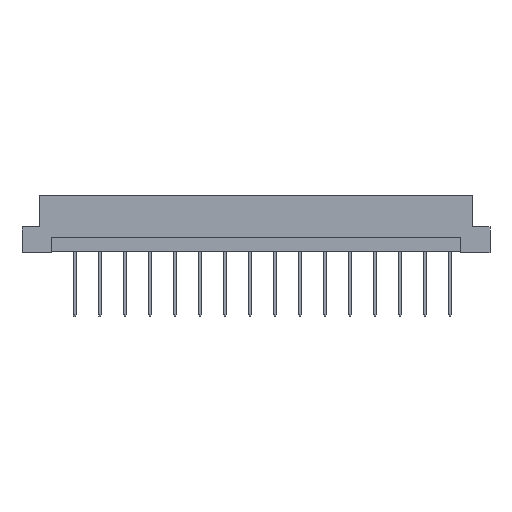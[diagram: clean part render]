
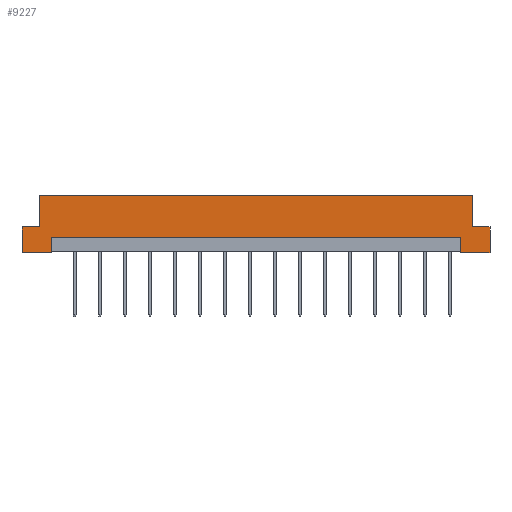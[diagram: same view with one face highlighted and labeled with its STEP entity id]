
A CAD part, front view. The second image highlights one B-rep face of the part: STEP entity #9227.
In plain terms, the highlighted planar face has unit normal (0, -1, 0).
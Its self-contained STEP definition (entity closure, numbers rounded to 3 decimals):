
#10 = VECTOR ( 'NONE', #4077, 1000. ) ;
#165 = VECTOR ( 'NONE', #2074, 1000. ) ;
#184 = CARTESIAN_POINT ( 'NONE',  ( 47.5, -4.3, 11.6 ) ) ;
#233 = VERTEX_POINT ( 'NONE', #4532 ) ;
#282 = EDGE_LOOP ( 'NONE', ( #6928, #5848, #4590, #3941, #6596, #9428, #8726, #10331, #349, #11098, #11080, #9771 ) ) ;
#314 = DIRECTION ( 'NONE',  ( 0., 0., -1. ) ) ;
#349 = ORIENTED_EDGE ( 'NONE', *, *, #6792, .F. ) ;
#429 = CARTESIAN_POINT ( 'NONE',  ( -41.6, -4.3, 0.2 ) ) ;
#440 = VERTEX_POINT ( 'NONE', #8201 ) ;
#538 = CARTESIAN_POINT ( 'NONE',  ( 41.6, -4.3, 0.2 ) ) ;
#577 = CARTESIAN_POINT ( 'NONE',  ( -44., -4.3, 5.2 ) ) ;
#586 = CARTESIAN_POINT ( 'NONE',  ( 47.5, -4.3, 11.6 ) ) ;
#843 = CARTESIAN_POINT ( 'NONE',  ( -47.5, -4.3, 0. ) ) ;
#1109 = DIRECTION ( 'NONE',  ( 1., 0., 0. ) ) ;
#1149 = CARTESIAN_POINT ( 'NONE',  ( 44., -4.3, 5.2 ) ) ;
#1509 = LINE ( 'NONE', #538, #3602 ) ;
#1613 = VERTEX_POINT ( 'NONE', #6684 ) ;
#1621 = VECTOR ( 'NONE', #2677, 1000. ) ;
#2074 = DIRECTION ( 'NONE',  ( 0., 0., -1. ) ) ;
#2199 = LINE ( 'NONE', #586, #10 ) ;
#2232 = CARTESIAN_POINT ( 'NONE',  ( 47.5, -4.3, 11.6 ) ) ;
#2236 = EDGE_CURVE ( 'NONE', #2378, #440, #11209, .T. ) ;
#2378 = VERTEX_POINT ( 'NONE', #7306 ) ;
#2518 = VECTOR ( 'NONE', #5658, 1000. ) ;
#2624 = VECTOR ( 'NONE', #4190, 1000. ) ;
#2677 = DIRECTION ( 'NONE',  ( 1., 0., 0. ) ) ;
#2834 = PLANE ( 'NONE',  #3171 ) ;
#2908 = LINE ( 'NONE', #429, #9891 ) ;
#3005 = DIRECTION ( 'NONE',  ( 0., 1., 0. ) ) ;
#3020 = VECTOR ( 'NONE', #5967, 1000. ) ;
#3037 = LINE ( 'NONE', #6526, #2518 ) ;
#3171 = AXIS2_PLACEMENT_3D ( 'NONE', #184, #3005, #5567 ) ;
#3565 = CARTESIAN_POINT ( 'NONE',  ( -41.6, -4.3, 3. ) ) ;
#3579 = VERTEX_POINT ( 'NONE', #4504 ) ;
#3602 = VECTOR ( 'NONE', #4996, 1000. ) ;
#3723 = VERTEX_POINT ( 'NONE', #4557 ) ;
#3771 = EDGE_CURVE ( 'NONE', #3579, #233, #2908, .T. ) ;
#3941 = ORIENTED_EDGE ( 'NONE', *, *, #4196, .F. ) ;
#4077 = DIRECTION ( 'NONE',  ( 0., 0., -1. ) ) ;
#4190 = DIRECTION ( 'NONE',  ( 1., 0., 0. ) ) ;
#4196 = EDGE_CURVE ( 'NONE', #3723, #440, #2199, .T. ) ;
#4491 = EDGE_CURVE ( 'NONE', #1613, #8023, #8034, .T. ) ;
#4504 = CARTESIAN_POINT ( 'NONE',  ( -41.6, -4.3, 3. ) ) ;
#4532 = CARTESIAN_POINT ( 'NONE',  ( -41.6, -4.3, 0. ) ) ;
#4543 = FACE_OUTER_BOUND ( 'NONE', #282, .T. ) ;
#4557 = CARTESIAN_POINT ( 'NONE',  ( 47.5, -4.3, 5.2 ) ) ;
#4590 = ORIENTED_EDGE ( 'NONE', *, *, #2236, .T. ) ;
#4996 = DIRECTION ( 'NONE',  ( 0., 0., 1. ) ) ;
#5567 = DIRECTION ( 'NONE',  ( -1., 0., 0. ) ) ;
#5658 = DIRECTION ( 'NONE',  ( 1., 0., 0. ) ) ;
#5783 = VECTOR ( 'NONE', #1109, 1000. ) ;
#5848 = ORIENTED_EDGE ( 'NONE', *, *, #6618, .F. ) ;
#5935 = VERTEX_POINT ( 'NONE', #577 ) ;
#5967 = DIRECTION ( 'NONE',  ( 1., 0., 0. ) ) ;
#6159 = CARTESIAN_POINT ( 'NONE',  ( 47.5, -4.3, 0. ) ) ;
#6364 = VECTOR ( 'NONE', #8271, 1000. ) ;
#6526 = CARTESIAN_POINT ( 'NONE',  ( 47.5, -4.3, 5.2 ) ) ;
#6527 = LINE ( 'NONE', #2232, #7024 ) ;
#6596 = ORIENTED_EDGE ( 'NONE', *, *, #7493, .F. ) ;
#6618 = EDGE_CURVE ( 'NONE', #2378, #11106, #1509, .T. ) ;
#6684 = CARTESIAN_POINT ( 'NONE',  ( -47.5, -4.3, 5.2 ) ) ;
#6792 = EDGE_CURVE ( 'NONE', #1613, #5935, #9870, .T. ) ;
#6928 = ORIENTED_EDGE ( 'NONE', *, *, #10822, .T. ) ;
#6982 = VERTEX_POINT ( 'NONE', #10143 ) ;
#7024 = VECTOR ( 'NONE', #10246, 1000. ) ;
#7174 = CARTESIAN_POINT ( 'NONE',  ( -47.5, -4.3, 5.2 ) ) ;
#7306 = CARTESIAN_POINT ( 'NONE',  ( 41.6, -4.3, 0. ) ) ;
#7370 = CARTESIAN_POINT ( 'NONE',  ( -44., -4.3, 5.2 ) ) ;
#7493 = EDGE_CURVE ( 'NONE', #11012, #3723, #3037, .T. ) ;
#8023 = VERTEX_POINT ( 'NONE', #843 ) ;
#8034 = LINE ( 'NONE', #9911, #165 ) ;
#8173 = EDGE_CURVE ( 'NONE', #11012, #6982, #9127, .T. ) ;
#8201 = CARTESIAN_POINT ( 'NONE',  ( 47.5, -4.3, 0. ) ) ;
#8271 = DIRECTION ( 'NONE',  ( 0., 0., 1. ) ) ;
#8499 = VERTEX_POINT ( 'NONE', #10604 ) ;
#8726 = ORIENTED_EDGE ( 'NONE', *, *, #9753, .F. ) ;
#8884 = VECTOR ( 'NONE', #9947, 1000. ) ;
#8981 = EDGE_CURVE ( 'NONE', #5935, #8499, #10758, .T. ) ;
#9127 = LINE ( 'NONE', #10040, #6364 ) ;
#9227 = ADVANCED_FACE ( 'NONE', ( #4543 ), #2834, .F. ) ;
#9428 = ORIENTED_EDGE ( 'NONE', *, *, #8173, .T. ) ;
#9536 = EDGE_CURVE ( 'NONE', #8023, #233, #10548, .T. ) ;
#9753 = EDGE_CURVE ( 'NONE', #8499, #6982, #6527, .T. ) ;
#9771 = ORIENTED_EDGE ( 'NONE', *, *, #3771, .F. ) ;
#9870 = LINE ( 'NONE', #7174, #5783 ) ;
#9891 = VECTOR ( 'NONE', #314, 1000. ) ;
#9911 = CARTESIAN_POINT ( 'NONE',  ( -47.5, -4.3, 11.6 ) ) ;
#9947 = DIRECTION ( 'NONE',  ( 0., 0., 1. ) ) ;
#10040 = CARTESIAN_POINT ( 'NONE',  ( 44., -4.3, 5.2 ) ) ;
#10143 = CARTESIAN_POINT ( 'NONE',  ( 44., -4.3, 11.6 ) ) ;
#10187 = CARTESIAN_POINT ( 'NONE',  ( 41.6, -4.3, 3. ) ) ;
#10246 = DIRECTION ( 'NONE',  ( 1., 0., 0. ) ) ;
#10331 = ORIENTED_EDGE ( 'NONE', *, *, #8981, .F. ) ;
#10548 = LINE ( 'NONE', #11182, #2624 ) ;
#10604 = CARTESIAN_POINT ( 'NONE',  ( -44., -4.3, 11.6 ) ) ;
#10605 = LINE ( 'NONE', #3565, #3020 ) ;
#10758 = LINE ( 'NONE', #7370, #8884 ) ;
#10822 = EDGE_CURVE ( 'NONE', #3579, #11106, #10605, .T. ) ;
#11012 = VERTEX_POINT ( 'NONE', #1149 ) ;
#11080 = ORIENTED_EDGE ( 'NONE', *, *, #9536, .T. ) ;
#11098 = ORIENTED_EDGE ( 'NONE', *, *, #4491, .T. ) ;
#11106 = VERTEX_POINT ( 'NONE', #10187 ) ;
#11182 = CARTESIAN_POINT ( 'NONE',  ( 47.5, -4.3, 0. ) ) ;
#11209 = LINE ( 'NONE', #6159, #1621 ) ;
